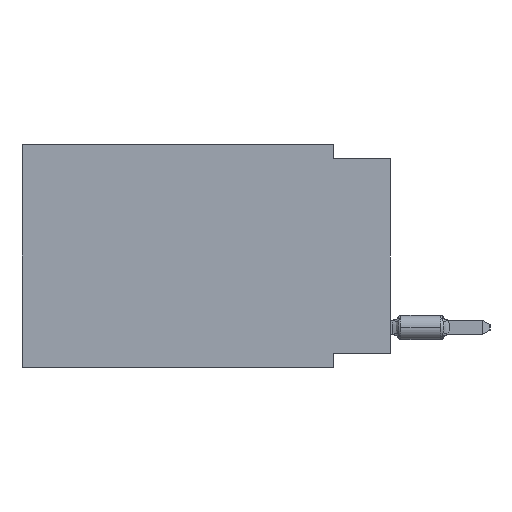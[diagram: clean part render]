
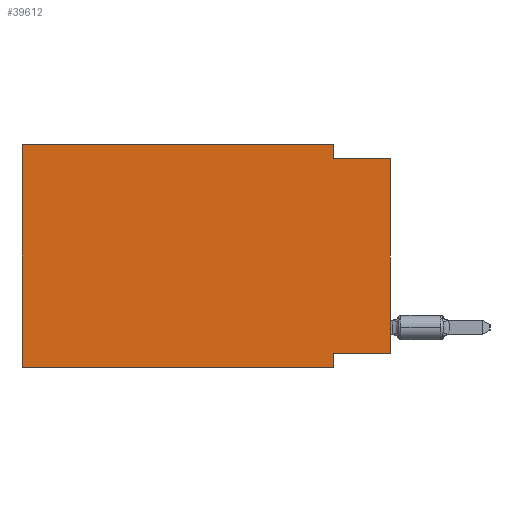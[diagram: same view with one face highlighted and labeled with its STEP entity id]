
A CAD part, left-side view. The second image highlights one B-rep face of the part: STEP entity #39612.
In plain terms, the highlighted planar face has unit normal (-1, 0, 0).
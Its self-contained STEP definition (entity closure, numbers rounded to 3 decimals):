
#283 = CARTESIAN_POINT ( 'NONE',  ( 0., 2.54, 0. ) ) ;
#356 = DIRECTION ( 'NONE',  ( 0., -1., 0. ) ) ;
#477 = VERTEX_POINT ( 'NONE', #19956 ) ;
#484 = VECTOR ( 'NONE', #25490, 1000. ) ;
#826 = LINE ( 'NONE', #29810, #42147 ) ;
#965 = ORIENTED_EDGE ( 'NONE', *, *, #43304, .T. ) ;
#1510 = VERTEX_POINT ( 'NONE', #33896 ) ;
#1594 = FACE_OUTER_BOUND ( 'NONE', #41051, .T. ) ;
#2589 = VECTOR ( 'NONE', #29111, 1000. ) ;
#3054 = AXIS2_PLACEMENT_3D ( 'NONE', #26556, #30573, #45350 ) ;
#3094 = VECTOR ( 'NONE', #13643, 1000. ) ;
#4496 = DIRECTION ( 'NONE',  ( 0., 1., 0. ) ) ;
#5516 = ORIENTED_EDGE ( 'NONE', *, *, #30369, .F. ) ;
#7785 = CARTESIAN_POINT ( 'NONE',  ( 0., 2.54, -9.906 ) ) ;
#8281 = CARTESIAN_POINT ( 'NONE',  ( 0., 0., -9.271 ) ) ;
#9280 = ORIENTED_EDGE ( 'NONE', *, *, #12305, .F. ) ;
#10622 = CARTESIAN_POINT ( 'NONE',  ( 0., 16.383, 0. ) ) ;
#10685 = ORIENTED_EDGE ( 'NONE', *, *, #22191, .F. ) ;
#12305 = EDGE_CURVE ( 'NONE', #23450, #1510, #30617, .T. ) ;
#12747 = PLANE ( 'NONE',  #3054 ) ;
#13577 = VERTEX_POINT ( 'NONE', #25332 ) ;
#13643 = DIRECTION ( 'NONE',  ( 0., 0., 1. ) ) ;
#15171 = CARTESIAN_POINT ( 'NONE',  ( 0., 16.383, -9.906 ) ) ;
#15665 = EDGE_CURVE ( 'NONE', #477, #13577, #39419, .T. ) ;
#16287 = EDGE_CURVE ( 'NONE', #26674, #21713, #18203, .T. ) ;
#18203 = LINE ( 'NONE', #32676, #2589 ) ;
#19866 = ORIENTED_EDGE ( 'NONE', *, *, #16287, .F. ) ;
#19956 = CARTESIAN_POINT ( 'NONE',  ( 0., 2.54, -0.635 ) ) ;
#21288 = CARTESIAN_POINT ( 'NONE',  ( 0., 2.54, -9.906 ) ) ;
#21713 = VERTEX_POINT ( 'NONE', #10622 ) ;
#22191 = EDGE_CURVE ( 'NONE', #21713, #44997, #826, .T. ) ;
#22430 = VECTOR ( 'NONE', #4496, 1000. ) ;
#22948 = EDGE_CURVE ( 'NONE', #44997, #477, #44012, .T. ) ;
#23450 = VERTEX_POINT ( 'NONE', #34593 ) ;
#24835 = CARTESIAN_POINT ( 'NONE',  ( 0., 0., 0. ) ) ;
#25332 = CARTESIAN_POINT ( 'NONE',  ( 0., 0., -0.635 ) ) ;
#25490 = DIRECTION ( 'NONE',  ( 0., 0., -1. ) ) ;
#26556 = CARTESIAN_POINT ( 'NONE',  ( 0., 16.383, 0. ) ) ;
#26674 = VERTEX_POINT ( 'NONE', #38461 ) ;
#28712 = DIRECTION ( 'NONE',  ( 0., -1., 0. ) ) ;
#29111 = DIRECTION ( 'NONE',  ( 0., 0., 1. ) ) ;
#29810 = CARTESIAN_POINT ( 'NONE',  ( 0., 16.383, 0. ) ) ;
#30369 = EDGE_CURVE ( 'NONE', #1510, #41366, #37501, .T. ) ;
#30572 = VECTOR ( 'NONE', #37509, 1000. ) ;
#30573 = DIRECTION ( 'NONE',  ( 1., 0., 0. ) ) ;
#30617 = LINE ( 'NONE', #8281, #22430 ) ;
#32676 = CARTESIAN_POINT ( 'NONE',  ( 0., 16.383, 0. ) ) ;
#33730 = ORIENTED_EDGE ( 'NONE', *, *, #46115, .T. ) ;
#33896 = CARTESIAN_POINT ( 'NONE',  ( 0., 2.54, -9.271 ) ) ;
#34593 = CARTESIAN_POINT ( 'NONE',  ( 0., 0., -9.271 ) ) ;
#36430 = ORIENTED_EDGE ( 'NONE', *, *, #15665, .F. ) ;
#37031 = DIRECTION ( 'NONE',  ( 0., 0., -1. ) ) ;
#37501 = LINE ( 'NONE', #7785, #42417 ) ;
#37509 = DIRECTION ( 'NONE',  ( 0., -1., 0. ) ) ;
#38017 = ORIENTED_EDGE ( 'NONE', *, *, #22948, .F. ) ;
#38256 = VECTOR ( 'NONE', #28712, 1000. ) ;
#38461 = CARTESIAN_POINT ( 'NONE',  ( 0., 16.383, -9.906 ) ) ;
#38857 = LINE ( 'NONE', #24835, #3094 ) ;
#39419 = LINE ( 'NONE', #46592, #38256 ) ;
#39612 = ADVANCED_FACE ( 'NONE', ( #1594 ), #12747, .F. ) ;
#41051 = EDGE_LOOP ( 'NONE', ( #965, #36430, #38017, #10685, #19866, #33730, #5516, #9280 ) ) ;
#41366 = VERTEX_POINT ( 'NONE', #21288 ) ;
#42147 = VECTOR ( 'NONE', #356, 1000. ) ;
#42378 = CARTESIAN_POINT ( 'NONE',  ( 0., 2.54, 0. ) ) ;
#42417 = VECTOR ( 'NONE', #37031, 1000. ) ;
#43304 = EDGE_CURVE ( 'NONE', #23450, #13577, #38857, .T. ) ;
#44012 = LINE ( 'NONE', #283, #484 ) ;
#44659 = LINE ( 'NONE', #15171, #30572 ) ;
#44997 = VERTEX_POINT ( 'NONE', #42378 ) ;
#45350 = DIRECTION ( 'NONE',  ( 0., 0., -1. ) ) ;
#46115 = EDGE_CURVE ( 'NONE', #26674, #41366, #44659, .T. ) ;
#46592 = CARTESIAN_POINT ( 'NONE',  ( 0., 0., -0.635 ) ) ;
